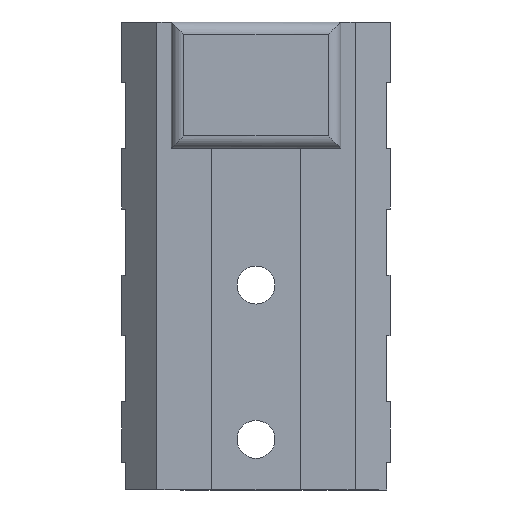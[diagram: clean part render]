
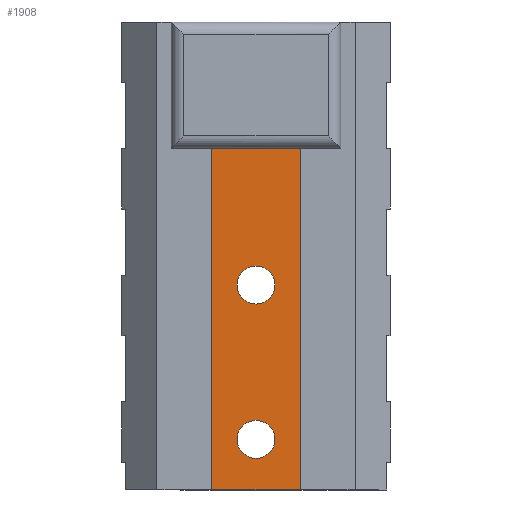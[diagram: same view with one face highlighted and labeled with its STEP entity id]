
A CAD part, front view. The second image highlights one B-rep face of the part: STEP entity #1908.
In plain terms, the highlighted planar face has unit normal (0, -1, 0).
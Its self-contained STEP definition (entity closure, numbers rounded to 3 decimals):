
#47 = CARTESIAN_POINT ( 'NONE',  ( -3.5, 1., -0.093 ) ) ;
#55 = CARTESIAN_POINT ( 'NONE',  ( 0., 1., -24.593 ) ) ;
#128 = AXIS2_PLACEMENT_3D ( 'NONE', #2045, #931, #2739 ) ;
#194 = CIRCLE ( 'NONE', #128, 1.5 ) ;
#195 = EDGE_LOOP ( 'NONE', ( #2831, #1942 ) ) ;
#209 = DIRECTION ( 'NONE',  ( 1., 0., 0. ) ) ;
#305 = EDGE_CURVE ( 'NONE', #2495, #2700, #922, .T. ) ;
#340 = ORIENTED_EDGE ( 'NONE', *, *, #856, .F. ) ;
#356 = DIRECTION ( 'NONE',  ( 0., 0., 1. ) ) ;
#357 = CIRCLE ( 'NONE', #1887, 1.5 ) ;
#425 = DIRECTION ( 'NONE',  ( 0., 1., 0. ) ) ;
#433 = CARTESIAN_POINT ( 'NONE',  ( 3.5, 1., -27.093 ) ) ;
#447 = PLANE ( 'NONE',  #1271 ) ;
#469 = EDGE_CURVE ( 'NONE', #1191, #1457, #846, .T. ) ;
#480 = DIRECTION ( 'NONE',  ( 0., 0., 1. ) ) ;
#532 = CARTESIAN_POINT ( 'NONE',  ( 3.5, 1., -27.093 ) ) ;
#544 = EDGE_CURVE ( 'NONE', #2495, #1425, #1780, .T. ) ;
#552 = FACE_OUTER_BOUND ( 'NONE', #797, .T. ) ;
#572 = CARTESIAN_POINT ( 'NONE',  ( 0., 1., -23.093 ) ) ;
#575 = AXIS2_PLACEMENT_3D ( 'NONE', #572, #2135, #1645 ) ;
#649 = VECTOR ( 'NONE', #209, 1000. ) ;
#666 = VERTEX_POINT ( 'NONE', #1491 ) ;
#690 = FACE_BOUND ( 'NONE', #195, .T. ) ;
#697 = AXIS2_PLACEMENT_3D ( 'NONE', #1922, #1242, #356 ) ;
#704 = LINE ( 'NONE', #47, #1898 ) ;
#743 = CARTESIAN_POINT ( 'NONE',  ( -3.5, 1., -27.093 ) ) ;
#797 = EDGE_LOOP ( 'NONE', ( #2264, #1413, #2792, #340 ) ) ;
#846 = CIRCLE ( 'NONE', #575, 1.5 ) ;
#856 = EDGE_CURVE ( 'NONE', #2700, #1040, #704, .T. ) ;
#879 = CIRCLE ( 'NONE', #697, 1.5 ) ;
#922 = LINE ( 'NONE', #743, #1473 ) ;
#931 = DIRECTION ( 'NONE',  ( 0., 1., 0. ) ) ;
#1040 = VERTEX_POINT ( 'NONE', #1205 ) ;
#1103 = CARTESIAN_POINT ( 'NONE',  ( -10.605, 1., -27.093 ) ) ;
#1178 = DIRECTION ( 'NONE',  ( -1., 0., 0. ) ) ;
#1191 = VERTEX_POINT ( 'NONE', #2387 ) ;
#1205 = CARTESIAN_POINT ( 'NONE',  ( -3.5, 1., -0.093 ) ) ;
#1216 = ORIENTED_EDGE ( 'NONE', *, *, #2040, .T. ) ;
#1242 = DIRECTION ( 'NONE',  ( 0., 1., 0. ) ) ;
#1271 = AXIS2_PLACEMENT_3D ( 'NONE', #1103, #425, #1329 ) ;
#1329 = DIRECTION ( 'NONE',  ( 0., 0., 1. ) ) ;
#1360 = CARTESIAN_POINT ( 'NONE',  ( 3.5, 1., -0.093 ) ) ;
#1413 = ORIENTED_EDGE ( 'NONE', *, *, #544, .T. ) ;
#1425 = VERTEX_POINT ( 'NONE', #1360 ) ;
#1449 = ORIENTED_EDGE ( 'NONE', *, *, #2855, .T. ) ;
#1457 = VERTEX_POINT ( 'NONE', #55 ) ;
#1473 = VECTOR ( 'NONE', #1178, 1000. ) ;
#1491 = CARTESIAN_POINT ( 'NONE',  ( 0., 1., -9.393 ) ) ;
#1593 = EDGE_CURVE ( 'NONE', #1457, #1191, #194, .T. ) ;
#1602 = CARTESIAN_POINT ( 'NONE',  ( -3.5, 1., -27.093 ) ) ;
#1645 = DIRECTION ( 'NONE',  ( 0., 0., 1. ) ) ;
#1676 = DIRECTION ( 'NONE',  ( 0., 0., 1. ) ) ;
#1773 = CARTESIAN_POINT ( 'NONE',  ( -10.605, 1., -0.093 ) ) ;
#1780 = LINE ( 'NONE', #532, #2080 ) ;
#1813 = DIRECTION ( 'NONE',  ( 0., 0., 1. ) ) ;
#1832 = CARTESIAN_POINT ( 'NONE',  ( 0., 1., -10.893 ) ) ;
#1887 = AXIS2_PLACEMENT_3D ( 'NONE', #1832, #2247, #1813 ) ;
#1898 = VECTOR ( 'NONE', #480, 1000. ) ;
#1908 = ADVANCED_FACE ( 'NONE', ( #690, #1989, #552 ), #447, .F. ) ;
#1922 = CARTESIAN_POINT ( 'NONE',  ( 0., 1., -10.893 ) ) ;
#1942 = ORIENTED_EDGE ( 'NONE', *, *, #469, .T. ) ;
#1989 = FACE_BOUND ( 'NONE', #2390, .T. ) ;
#2005 = LINE ( 'NONE', #1773, #649 ) ;
#2040 = EDGE_CURVE ( 'NONE', #666, #2164, #357, .T. ) ;
#2045 = CARTESIAN_POINT ( 'NONE',  ( 0., 1., -23.093 ) ) ;
#2080 = VECTOR ( 'NONE', #1676, 1000. ) ;
#2135 = DIRECTION ( 'NONE',  ( 0., 1., 0. ) ) ;
#2164 = VERTEX_POINT ( 'NONE', #2780 ) ;
#2247 = DIRECTION ( 'NONE',  ( 0., 1., 0. ) ) ;
#2264 = ORIENTED_EDGE ( 'NONE', *, *, #305, .F. ) ;
#2387 = CARTESIAN_POINT ( 'NONE',  ( 0., 1., -21.593 ) ) ;
#2390 = EDGE_LOOP ( 'NONE', ( #1449, #1216 ) ) ;
#2495 = VERTEX_POINT ( 'NONE', #433 ) ;
#2540 = EDGE_CURVE ( 'NONE', #1040, #1425, #2005, .T. ) ;
#2700 = VERTEX_POINT ( 'NONE', #1602 ) ;
#2739 = DIRECTION ( 'NONE',  ( 0., 0., 1. ) ) ;
#2780 = CARTESIAN_POINT ( 'NONE',  ( 0., 1., -12.394 ) ) ;
#2792 = ORIENTED_EDGE ( 'NONE', *, *, #2540, .F. ) ;
#2831 = ORIENTED_EDGE ( 'NONE', *, *, #1593, .T. ) ;
#2855 = EDGE_CURVE ( 'NONE', #2164, #666, #879, .T. ) ;
